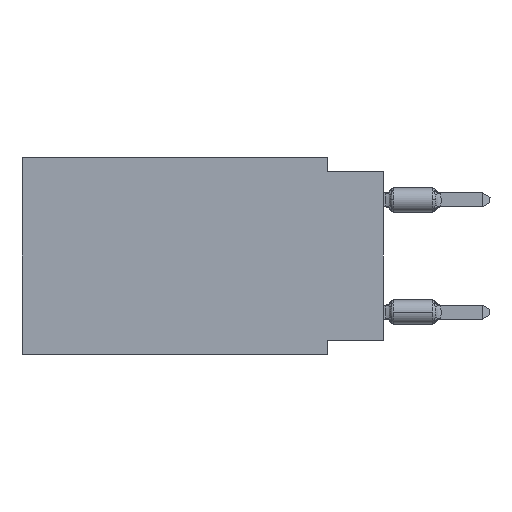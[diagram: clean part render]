
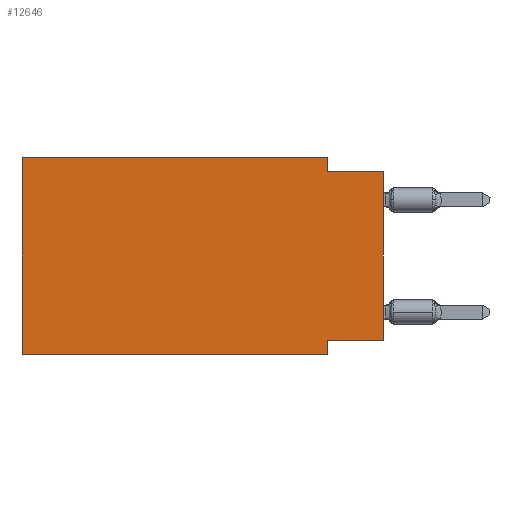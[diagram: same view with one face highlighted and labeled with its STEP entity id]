
A CAD part, left-side view. The second image highlights one B-rep face of the part: STEP entity #12646.
In plain terms, the highlighted planar face has unit normal (-1, 0, 0).
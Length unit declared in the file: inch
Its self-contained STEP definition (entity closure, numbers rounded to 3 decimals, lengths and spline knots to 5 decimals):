
#218 = LINE ( 'NONE', #2319, #11155 ) ;
#514 = EDGE_CURVE ( 'NONE', #20905, #7491, #8829, .T. ) ;
#566 = LINE ( 'NONE', #18895, #13527 ) ;
#656 = VERTEX_POINT ( 'NONE', #22675 ) ;
#943 = DIRECTION ( 'NONE',  ( 0., 0., -1. ) ) ;
#1792 = PLANE ( 'NONE',  #3010 ) ;
#1858 = ORIENTED_EDGE ( 'NONE', *, *, #7462, .F. ) ;
#2319 = CARTESIAN_POINT ( 'NONE',  ( 0., 0., -0.325 ) ) ;
#2365 = VERTEX_POINT ( 'NONE', #12672 ) ;
#3010 = AXIS2_PLACEMENT_3D ( 'NONE', #13075, #16988, #26639 ) ;
#4344 = DIRECTION ( 'NONE',  ( 0., 0., 1. ) ) ;
#4537 = LINE ( 'NONE', #25360, #26425 ) ;
#4793 = VERTEX_POINT ( 'NONE', #27526 ) ;
#4962 = CARTESIAN_POINT ( 'NONE',  ( 0., 0.1, 0. ) ) ;
#5116 = EDGE_CURVE ( 'NONE', #20905, #4793, #14994, .T. ) ;
#5190 = VERTEX_POINT ( 'NONE', #29074 ) ;
#6287 = VECTOR ( 'NONE', #943, 39.37008 ) ;
#6533 = VECTOR ( 'NONE', #13723, 39.37008 ) ;
#6641 = DIRECTION ( 'NONE',  ( 0., 1., 0. ) ) ;
#6691 = ORIENTED_EDGE ( 'NONE', *, *, #5116, .T. ) ;
#6996 = ORIENTED_EDGE ( 'NONE', *, *, #10883, .F. ) ;
#7276 = DIRECTION ( 'NONE',  ( 0., 0., -1. ) ) ;
#7462 = EDGE_CURVE ( 'NONE', #656, #13920, #12240, .T. ) ;
#7491 = VERTEX_POINT ( 'NONE', #13126 ) ;
#8829 = LINE ( 'NONE', #26990, #20152 ) ;
#9128 = LINE ( 'NONE', #20008, #17380 ) ;
#9296 = ORIENTED_EDGE ( 'NONE', *, *, #19354, .F. ) ;
#10883 = EDGE_CURVE ( 'NONE', #13920, #5190, #9128, .T. ) ;
#11155 = VECTOR ( 'NONE', #6641, 39.37008 ) ;
#11443 = ORIENTED_EDGE ( 'NONE', *, *, #27872, .F. ) ;
#12240 = LINE ( 'NONE', #4962, #6287 ) ;
#12646 = ADVANCED_FACE ( 'NONE', ( #17548 ), #1792, .F. ) ;
#12672 = CARTESIAN_POINT ( 'NONE',  ( 0., 0., -0.325 ) ) ;
#13075 = CARTESIAN_POINT ( 'NONE',  ( 0., 0.645, 0. ) ) ;
#13126 = CARTESIAN_POINT ( 'NONE',  ( 0., 0.645, 0. ) ) ;
#13527 = VECTOR ( 'NONE', #7276, 39.37008 ) ;
#13723 = DIRECTION ( 'NONE',  ( 0., -1., 0. ) ) ;
#13920 = VERTEX_POINT ( 'NONE', #19838 ) ;
#14031 = CARTESIAN_POINT ( 'NONE',  ( 0., 0.645, 0. ) ) ;
#14994 = LINE ( 'NONE', #24764, #6533 ) ;
#16988 = DIRECTION ( 'NONE',  ( 1., 0., 0. ) ) ;
#17380 = VECTOR ( 'NONE', #20158, 39.37008 ) ;
#17548 = FACE_OUTER_BOUND ( 'NONE', #28575, .T. ) ;
#17793 = ORIENTED_EDGE ( 'NONE', *, *, #21282, .F. ) ;
#17814 = VECTOR ( 'NONE', #23585, 39.37008 ) ;
#18824 = CARTESIAN_POINT ( 'NONE',  ( 0., 0.1, -0.325 ) ) ;
#18895 = CARTESIAN_POINT ( 'NONE',  ( 0., 0.1, -0.35 ) ) ;
#19354 = EDGE_CURVE ( 'NONE', #29217, #4793, #566, .T. ) ;
#19838 = CARTESIAN_POINT ( 'NONE',  ( 0., 0.1, -0.025 ) ) ;
#20008 = CARTESIAN_POINT ( 'NONE',  ( 0., 0., -0.025 ) ) ;
#20152 = VECTOR ( 'NONE', #4344, 39.37008 ) ;
#20158 = DIRECTION ( 'NONE',  ( 0., -1., 0. ) ) ;
#20905 = VERTEX_POINT ( 'NONE', #23651 ) ;
#21282 = EDGE_CURVE ( 'NONE', #2365, #29217, #218, .T. ) ;
#22675 = CARTESIAN_POINT ( 'NONE',  ( 0., 0.1, 0. ) ) ;
#23157 = DIRECTION ( 'NONE',  ( 0., 0., 1. ) ) ;
#23585 = DIRECTION ( 'NONE',  ( 0., -1., 0. ) ) ;
#23651 = CARTESIAN_POINT ( 'NONE',  ( 0., 0.645, -0.35 ) ) ;
#24764 = CARTESIAN_POINT ( 'NONE',  ( 0., 0.645, -0.35 ) ) ;
#25360 = CARTESIAN_POINT ( 'NONE',  ( 0., 0., 0. ) ) ;
#25786 = LINE ( 'NONE', #14031, #17814 ) ;
#25806 = ORIENTED_EDGE ( 'NONE', *, *, #514, .F. ) ;
#26425 = VECTOR ( 'NONE', #23157, 39.37008 ) ;
#26631 = ORIENTED_EDGE ( 'NONE', *, *, #29205, .T. ) ;
#26639 = DIRECTION ( 'NONE',  ( 0., 0., -1. ) ) ;
#26990 = CARTESIAN_POINT ( 'NONE',  ( 0., 0.645, 0. ) ) ;
#27526 = CARTESIAN_POINT ( 'NONE',  ( 0., 0.1, -0.35 ) ) ;
#27872 = EDGE_CURVE ( 'NONE', #7491, #656, #25786, .T. ) ;
#28575 = EDGE_LOOP ( 'NONE', ( #26631, #6996, #1858, #11443, #25806, #6691, #9296, #17793 ) ) ;
#29074 = CARTESIAN_POINT ( 'NONE',  ( 0., 0., -0.025 ) ) ;
#29205 = EDGE_CURVE ( 'NONE', #2365, #5190, #4537, .T. ) ;
#29217 = VERTEX_POINT ( 'NONE', #18824 ) ;
